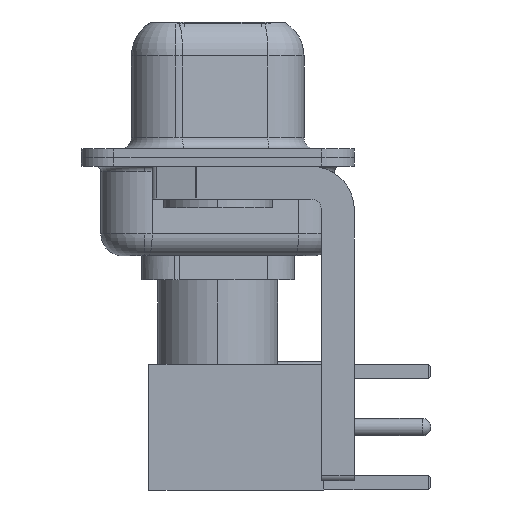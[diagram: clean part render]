
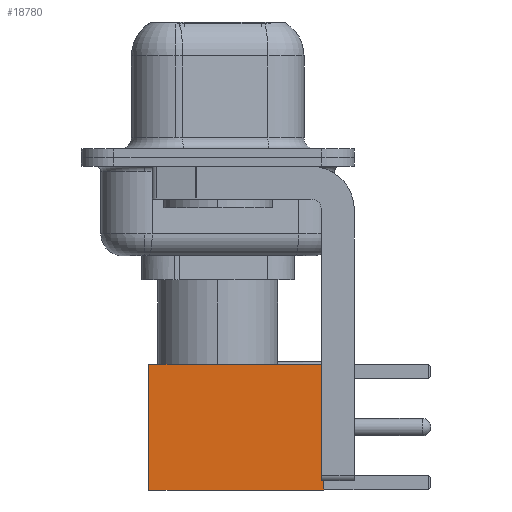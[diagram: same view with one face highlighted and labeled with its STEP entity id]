
A CAD part, left-side view. The second image highlights one B-rep face of the part: STEP entity #18780.
In plain terms, the highlighted face is planar.
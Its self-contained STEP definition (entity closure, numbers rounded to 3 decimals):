
#261 = DIRECTION ( 'NONE',  ( 0., 1., 0. ) ) ;
#444 = CARTESIAN_POINT ( 'NONE',  ( 2.875, 2.875, 0. ) ) ;
#494 = FACE_OUTER_BOUND ( 'NONE', #2083, .T. ) ;
#682 = CARTESIAN_POINT ( 'NONE',  ( 0., 2.875, 0. ) ) ;
#790 = LINE ( 'NONE', #682, #8843 ) ;
#952 = LINE ( 'NONE', #15453, #21767 ) ;
#1915 = VERTEX_POINT ( 'NONE', #5073 ) ;
#2083 = EDGE_LOOP ( 'NONE', ( #8440, #7506, #12581, #22146 ) ) ;
#2295 = CARTESIAN_POINT ( 'NONE',  ( -2.875, 2.875, 0. ) ) ;
#3636 = VERTEX_POINT ( 'NONE', #444 ) ;
#3757 = EDGE_CURVE ( 'NONE', #3636, #3842, #790, .T. ) ;
#3842 = VERTEX_POINT ( 'NONE', #4251 ) ;
#4251 = CARTESIAN_POINT ( 'NONE',  ( -2.875, 2.875, 0. ) ) ;
#4703 = EDGE_CURVE ( 'NONE', #10041, #1915, #952, .T. ) ;
#5073 = CARTESIAN_POINT ( 'NONE',  ( -2.875, 2.875, 8. ) ) ;
#5336 = AXIS2_PLACEMENT_3D ( 'NONE', #7758, #261, #5625 ) ;
#5625 = DIRECTION ( 'NONE',  ( 0., 0., 1. ) ) ;
#7506 = ORIENTED_EDGE ( 'NONE', *, *, #3757, .T. ) ;
#7611 = CARTESIAN_POINT ( 'NONE',  ( 2.875, 2.875, 8. ) ) ;
#7758 = CARTESIAN_POINT ( 'NONE',  ( 2.875, 2.875, 0. ) ) ;
#8440 = ORIENTED_EDGE ( 'NONE', *, *, #17007, .T. ) ;
#8843 = VECTOR ( 'NONE', #20780, 1000. ) ;
#9568 = DIRECTION ( 'NONE',  ( 0., 0., -1. ) ) ;
#10041 = VERTEX_POINT ( 'NONE', #7611 ) ;
#11018 = VECTOR ( 'NONE', #9568, 1000. ) ;
#11550 = DIRECTION ( 'NONE',  ( -1., 0., 0. ) ) ;
#11670 = CARTESIAN_POINT ( 'NONE',  ( 2.875, 2.875, 0. ) ) ;
#11883 = PLANE ( 'NONE',  #5336 ) ;
#12581 = ORIENTED_EDGE ( 'NONE', *, *, #18340, .F. ) ;
#13481 = LINE ( 'NONE', #2295, #11018 ) ;
#15453 = CARTESIAN_POINT ( 'NONE',  ( 0., 2.875, 8. ) ) ;
#17007 = EDGE_CURVE ( 'NONE', #10041, #3636, #22471, .T. ) ;
#18340 = EDGE_CURVE ( 'NONE', #1915, #3842, #13481, .T. ) ;
#18780 = ADVANCED_FACE ( 'NONE', ( #494 ), #11883, .T. ) ;
#20047 = VECTOR ( 'NONE', #20705, 1000. ) ;
#20705 = DIRECTION ( 'NONE',  ( 0., 0., -1. ) ) ;
#20780 = DIRECTION ( 'NONE',  ( -1., 0., 0. ) ) ;
#21767 = VECTOR ( 'NONE', #11550, 1000. ) ;
#22146 = ORIENTED_EDGE ( 'NONE', *, *, #4703, .F. ) ;
#22471 = LINE ( 'NONE', #11670, #20047 ) ;
